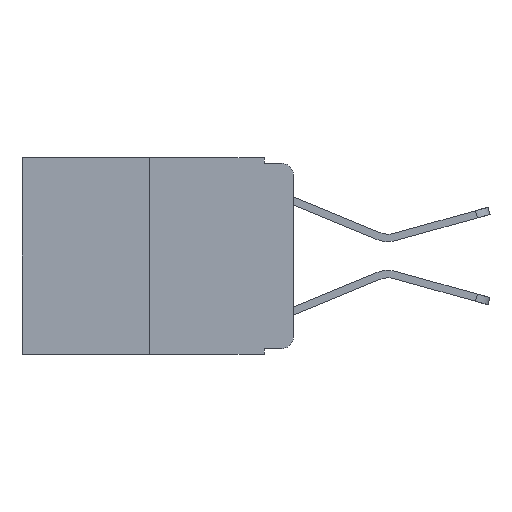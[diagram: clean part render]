
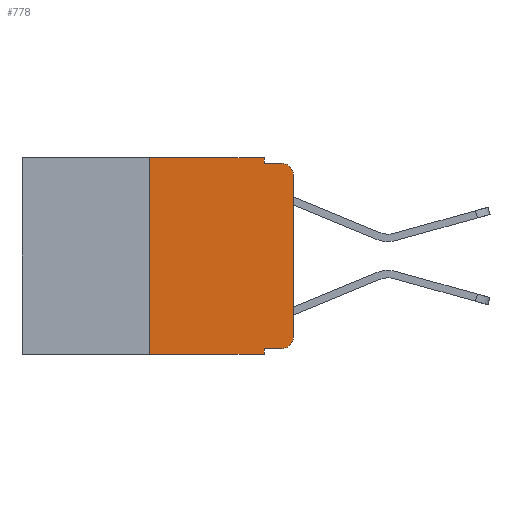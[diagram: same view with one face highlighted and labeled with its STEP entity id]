
A CAD part, left-side view. The second image highlights one B-rep face of the part: STEP entity #778.
In plain terms, the highlighted planar face has unit normal (-1, 0, 0).
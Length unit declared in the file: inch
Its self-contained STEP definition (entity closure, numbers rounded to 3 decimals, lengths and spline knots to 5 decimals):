
#166 = DIRECTION ( 'NONE',  ( 0., 0., -1. ) ) ;
#210 = ORIENTED_EDGE ( 'NONE', *, *, #5451, .T. ) ;
#431 = VECTOR ( 'NONE', #17143, 39.37008 ) ;
#778 = ADVANCED_FACE ( 'NONE', ( #2266 ), #9404, .F. ) ;
#979 = DIRECTION ( 'NONE',  ( 0., 0., 1. ) ) ;
#1012 = LINE ( 'NONE', #20688, #431 ) ;
#1233 = CARTESIAN_POINT ( 'NONE',  ( 0., 0.051, 0. ) ) ;
#1262 = EDGE_CURVE ( 'NONE', #12296, #21330, #15834, .T. ) ;
#1614 = EDGE_LOOP ( 'NONE', ( #21395, #14613, #17761, #18302, #6594, #2807, #14609, #19973, #3368, #210 ) ) ;
#1671 = CARTESIAN_POINT ( 'NONE',  ( 0., 0.051, -0.01 ) ) ;
#1689 = EDGE_CURVE ( 'NONE', #16593, #21098, #16938, .T. ) ;
#2266 = FACE_OUTER_BOUND ( 'NONE', #1614, .T. ) ;
#2749 = CARTESIAN_POINT ( 'NONE',  ( 0., 0.25, -0.343 ) ) ;
#2807 = ORIENTED_EDGE ( 'NONE', *, *, #1689, .F. ) ;
#3179 = VERTEX_POINT ( 'NONE', #16568 ) ;
#3240 = LINE ( 'NONE', #17297, #12513 ) ;
#3368 = ORIENTED_EDGE ( 'NONE', *, *, #13679, .T. ) ;
#3450 = CIRCLE ( 'NONE', #19549, 0.02 ) ;
#3537 = CARTESIAN_POINT ( 'NONE',  ( 0., 0.051, -0.333 ) ) ;
#3770 = VERTEX_POINT ( 'NONE', #8951 ) ;
#3897 = VERTEX_POINT ( 'NONE', #12975 ) ;
#4315 = VERTEX_POINT ( 'NONE', #10460 ) ;
#4801 = CARTESIAN_POINT ( 'NONE',  ( 0., 0.02, -0.313 ) ) ;
#4974 = CARTESIAN_POINT ( 'NONE',  ( 0., 0.473, 0. ) ) ;
#5201 = VECTOR ( 'NONE', #979, 39.37008 ) ;
#5422 = EDGE_CURVE ( 'NONE', #3179, #3897, #15010, .T. ) ;
#5451 = EDGE_CURVE ( 'NONE', #21191, #3179, #14444, .T. ) ;
#5644 = DIRECTION ( 'NONE',  ( -1., 0., 0. ) ) ;
#6594 = ORIENTED_EDGE ( 'NONE', *, *, #20154, .F. ) ;
#6679 = DIRECTION ( 'NONE',  ( 0., 0., -1. ) ) ;
#6715 = CARTESIAN_POINT ( 'NONE',  ( 0., 0.25, 0. ) ) ;
#6846 = DIRECTION ( 'NONE',  ( 0., 0., -1. ) ) ;
#7929 = EDGE_CURVE ( 'NONE', #16593, #3770, #1012, .T. ) ;
#8169 = DIRECTION ( 'NONE',  ( 0., -1., 0. ) ) ;
#8705 = CARTESIAN_POINT ( 'NONE',  ( 0., 0.051, 0. ) ) ;
#8853 = VECTOR ( 'NONE', #23225, 39.37008 ) ;
#8951 = CARTESIAN_POINT ( 'NONE',  ( 0., 0.051, -0.343 ) ) ;
#9404 = PLANE ( 'NONE',  #17851 ) ;
#9833 = EDGE_CURVE ( 'NONE', #15073, #3770, #18184, .T. ) ;
#10431 = DIRECTION ( 'NONE',  ( 0., 0., 1. ) ) ;
#10460 = CARTESIAN_POINT ( 'NONE',  ( 0., 0.051, 0. ) ) ;
#10516 = CARTESIAN_POINT ( 'NONE',  ( 0., 0.02, -0.01 ) ) ;
#11043 = AXIS2_PLACEMENT_3D ( 'NONE', #4801, #17654, #6679 ) ;
#11215 = CARTESIAN_POINT ( 'NONE',  ( 0., 0.051, -0.01 ) ) ;
#11266 = DIRECTION ( 'NONE',  ( 1., 0., 0. ) ) ;
#12296 = VERTEX_POINT ( 'NONE', #11215 ) ;
#12513 = VECTOR ( 'NONE', #8169, 39.37008 ) ;
#12975 = CARTESIAN_POINT ( 'NONE',  ( 0., 0., -0.03 ) ) ;
#13679 = EDGE_CURVE ( 'NONE', #15073, #21191, #3240, .T. ) ;
#13751 = LINE ( 'NONE', #4974, #8853 ) ;
#14320 = LINE ( 'NONE', #1233, #23323 ) ;
#14444 = CIRCLE ( 'NONE', #11043, 0.02 ) ;
#14594 = DIRECTION ( 'NONE',  ( 0., -1., 0. ) ) ;
#14609 = ORIENTED_EDGE ( 'NONE', *, *, #7929, .T. ) ;
#14613 = ORIENTED_EDGE ( 'NONE', *, *, #17325, .T. ) ;
#15010 = LINE ( 'NONE', #17510, #5201 ) ;
#15073 = VERTEX_POINT ( 'NONE', #3537 ) ;
#15263 = VECTOR ( 'NONE', #14594, 39.37008 ) ;
#15834 = LINE ( 'NONE', #1671, #15263 ) ;
#16010 = DIRECTION ( 'NONE',  ( 0., 0., -1. ) ) ;
#16568 = CARTESIAN_POINT ( 'NONE',  ( 0., 0., -0.313 ) ) ;
#16593 = VERTEX_POINT ( 'NONE', #2749 ) ;
#16658 = CARTESIAN_POINT ( 'NONE',  ( 0., 0.02, -0.03 ) ) ;
#16938 = LINE ( 'NONE', #6715, #21164 ) ;
#17143 = DIRECTION ( 'NONE',  ( 0., -1., 0. ) ) ;
#17297 = CARTESIAN_POINT ( 'NONE',  ( 0., 0.051, -0.333 ) ) ;
#17325 = EDGE_CURVE ( 'NONE', #3897, #21330, #3450, .T. ) ;
#17510 = CARTESIAN_POINT ( 'NONE',  ( 0., 0., 0. ) ) ;
#17654 = DIRECTION ( 'NONE',  ( -1., 0., 0. ) ) ;
#17761 = ORIENTED_EDGE ( 'NONE', *, *, #1262, .F. ) ;
#17851 = AXIS2_PLACEMENT_3D ( 'NONE', #22110, #11266, #166 ) ;
#18184 = LINE ( 'NONE', #8705, #22397 ) ;
#18302 = ORIENTED_EDGE ( 'NONE', *, *, #20133, .F. ) ;
#18455 = DIRECTION ( 'NONE',  ( 0., 0., -1. ) ) ;
#19190 = CARTESIAN_POINT ( 'NONE',  ( 0., 0.02, -0.333 ) ) ;
#19549 = AXIS2_PLACEMENT_3D ( 'NONE', #16658, #5644, #18455 ) ;
#19973 = ORIENTED_EDGE ( 'NONE', *, *, #9833, .F. ) ;
#20133 = EDGE_CURVE ( 'NONE', #4315, #12296, #14320, .T. ) ;
#20154 = EDGE_CURVE ( 'NONE', #21098, #4315, #13751, .T. ) ;
#20688 = CARTESIAN_POINT ( 'NONE',  ( 0., 0.473, -0.343 ) ) ;
#21098 = VERTEX_POINT ( 'NONE', #22558 ) ;
#21164 = VECTOR ( 'NONE', #10431, 39.37008 ) ;
#21191 = VERTEX_POINT ( 'NONE', #19190 ) ;
#21330 = VERTEX_POINT ( 'NONE', #10516 ) ;
#21395 = ORIENTED_EDGE ( 'NONE', *, *, #5422, .T. ) ;
#22110 = CARTESIAN_POINT ( 'NONE',  ( 0., 0.473, 0. ) ) ;
#22397 = VECTOR ( 'NONE', #6846, 39.37008 ) ;
#22558 = CARTESIAN_POINT ( 'NONE',  ( 0., 0.25, 0. ) ) ;
#23225 = DIRECTION ( 'NONE',  ( 0., -1., 0. ) ) ;
#23323 = VECTOR ( 'NONE', #16010, 39.37008 ) ;
